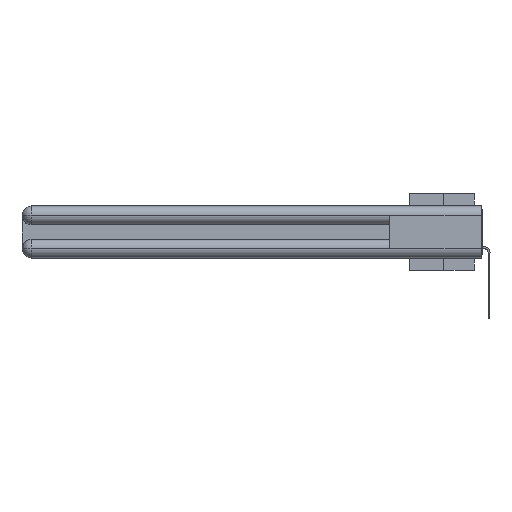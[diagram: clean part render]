
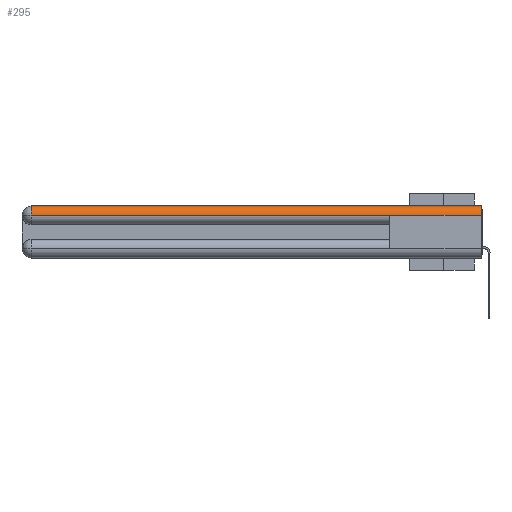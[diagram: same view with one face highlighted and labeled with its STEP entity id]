
A CAD part, left-side view. The second image highlights one B-rep face of the part: STEP entity #295.
In plain terms, the highlighted cylindrical face has radius 1.562 mm (diameter 3.124 mm), a partial arc.
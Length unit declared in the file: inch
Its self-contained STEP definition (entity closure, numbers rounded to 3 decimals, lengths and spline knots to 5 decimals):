
#295 = ADVANCED_FACE ( 'NONE', ( #9373 ), #14172, .T. ) ;
#859 = CARTESIAN_POINT ( 'NONE',  ( 0.0615, 0., -0.0615 ) ) ;
#2053 = LINE ( 'NONE', #4589, #24976 ) ;
#2328 = EDGE_CURVE ( 'NONE', #13435, #29247, #20046, .T. ) ;
#2379 = CARTESIAN_POINT ( 'NONE',  ( 0., 3., -0.0615 ) ) ;
#2917 = DIRECTION ( 'NONE',  ( 0., -1., 0. ) ) ;
#3444 = DIRECTION ( 'NONE',  ( 1., 0., 0. ) ) ;
#4353 = AXIS2_PLACEMENT_3D ( 'NONE', #5363, #21888, #12769 ) ;
#4589 = CARTESIAN_POINT ( 'NONE',  ( 0., 3., -0.0615 ) ) ;
#4742 = LINE ( 'NONE', #22077, #26189 ) ;
#5219 = DIRECTION ( 'NONE',  ( 0., 0., 1. ) ) ;
#5326 = CARTESIAN_POINT ( 'NONE',  ( 0.0615, 2.94, -0.0615 ) ) ;
#5363 = CARTESIAN_POINT ( 'NONE',  ( 0.0615, 0., -0.0615 ) ) ;
#5585 = EDGE_CURVE ( 'NONE', #22738, #13435, #4742, .T. ) ;
#7538 = DIRECTION ( 'NONE',  ( 0., -1., 0. ) ) ;
#8800 = LINE ( 'NONE', #2379, #12111 ) ;
#9373 = FACE_OUTER_BOUND ( 'NONE', #21815, .T. ) ;
#9541 = DIRECTION ( 'NONE',  ( 0., 1., 0. ) ) ;
#11498 = ORIENTED_EDGE ( 'NONE', *, *, #2328, .F. ) ;
#12111 = VECTOR ( 'NONE', #23682, 39.37008 ) ;
#12769 = DIRECTION ( 'NONE',  ( 0., 0., 1. ) ) ;
#13435 = VERTEX_POINT ( 'NONE', #30052 ) ;
#13792 = CIRCLE ( 'NONE', #20483, 0.0615 ) ;
#14172 = CYLINDRICAL_SURFACE ( 'NONE', #4353, 0.0615 ) ;
#14498 = CARTESIAN_POINT ( 'NONE',  ( 0., 0.6, -0.0615 ) ) ;
#14771 = ORIENTED_EDGE ( 'NONE', *, *, #26961, .F. ) ;
#15110 = DIRECTION ( 'NONE',  ( 0., -1., 0. ) ) ;
#18381 = EDGE_CURVE ( 'NONE', #26692, #27103, #8800, .T. ) ;
#19618 = ORIENTED_EDGE ( 'NONE', *, *, #18381, .T. ) ;
#20046 = CIRCLE ( 'NONE', #23430, 0.0615 ) ;
#20483 = AXIS2_PLACEMENT_3D ( 'NONE', #5326, #2917, #5219 ) ;
#21815 = EDGE_LOOP ( 'NONE', ( #25118, #28298, #19618, #14771, #11498 ) ) ;
#21888 = DIRECTION ( 'NONE',  ( 0., 1., 0. ) ) ;
#22077 = CARTESIAN_POINT ( 'NONE',  ( 0.0615, 0., 0. ) ) ;
#22738 = VERTEX_POINT ( 'NONE', #29967 ) ;
#23168 = EDGE_CURVE ( 'NONE', #22738, #26692, #13792, .T. ) ;
#23430 = AXIS2_PLACEMENT_3D ( 'NONE', #859, #15110, #3444 ) ;
#23682 = DIRECTION ( 'NONE',  ( 0., -1., 0. ) ) ;
#24926 = CARTESIAN_POINT ( 'NONE',  ( 0., 2.94, -0.0615 ) ) ;
#24976 = VECTOR ( 'NONE', #9541, 39.37008 ) ;
#25118 = ORIENTED_EDGE ( 'NONE', *, *, #5585, .F. ) ;
#26189 = VECTOR ( 'NONE', #7538, 39.37008 ) ;
#26692 = VERTEX_POINT ( 'NONE', #24926 ) ;
#26961 = EDGE_CURVE ( 'NONE', #29247, #27103, #2053, .T. ) ;
#27103 = VERTEX_POINT ( 'NONE', #14498 ) ;
#27993 = CARTESIAN_POINT ( 'NONE',  ( 0., 0., -0.0615 ) ) ;
#28298 = ORIENTED_EDGE ( 'NONE', *, *, #23168, .T. ) ;
#29247 = VERTEX_POINT ( 'NONE', #27993 ) ;
#29967 = CARTESIAN_POINT ( 'NONE',  ( 0.0615, 2.94, 0. ) ) ;
#30052 = CARTESIAN_POINT ( 'NONE',  ( 0.0615, 0., 0. ) ) ;
